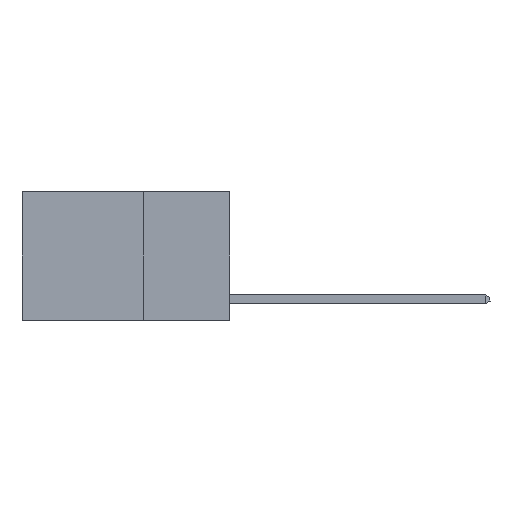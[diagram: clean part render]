
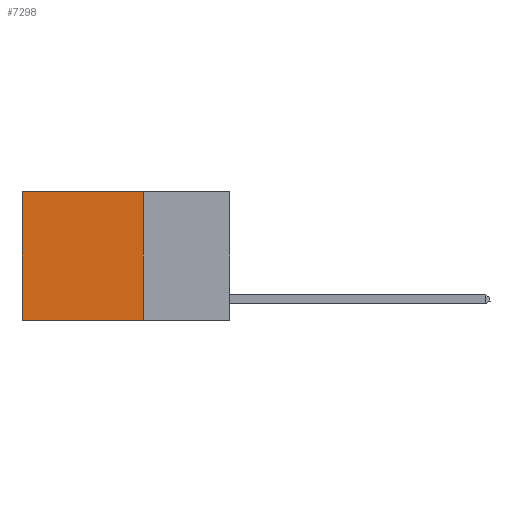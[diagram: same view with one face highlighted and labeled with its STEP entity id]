
A CAD part, left-side view. The second image highlights one B-rep face of the part: STEP entity #7298.
In plain terms, the highlighted planar face has unit normal (-1, 0, 0).
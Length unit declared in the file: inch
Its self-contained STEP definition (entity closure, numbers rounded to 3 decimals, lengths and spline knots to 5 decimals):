
#525 = EDGE_CURVE ( 'NONE', #13906, #12765, #7784, .T. ) ;
#599 = PLANE ( 'NONE',  #6531 ) ;
#750 = EDGE_CURVE ( 'NONE', #3400, #12765, #1172, .T. ) ;
#969 = VECTOR ( 'NONE', #12122, 39.37008 ) ;
#1172 = LINE ( 'NONE', #15113, #14037 ) ;
#1444 = EDGE_CURVE ( 'NONE', #3061, #13906, #5212, .T. ) ;
#1933 = DIRECTION ( 'NONE',  ( 1., 0., 0. ) ) ;
#2362 = VECTOR ( 'NONE', #7436, 39.37008 ) ;
#2688 = DIRECTION ( 'NONE',  ( 0., 0., -1. ) ) ;
#2980 = CARTESIAN_POINT ( 'NONE',  ( 0.2625, 0.6, 0. ) ) ;
#3061 = VERTEX_POINT ( 'NONE', #15967 ) ;
#3400 = VERTEX_POINT ( 'NONE', #2980 ) ;
#3490 = CARTESIAN_POINT ( 'NONE',  ( 0.2625, 0.6, -0.37 ) ) ;
#3659 = FACE_OUTER_BOUND ( 'NONE', #14649, .T. ) ;
#4446 = CARTESIAN_POINT ( 'NONE',  ( 0.2625, 0.25, -0.37 ) ) ;
#4913 = CARTESIAN_POINT ( 'NONE',  ( 0.2625, 0.25, 0. ) ) ;
#5131 = ORIENTED_EDGE ( 'NONE', *, *, #750, .T. ) ;
#5212 = LINE ( 'NONE', #10831, #14590 ) ;
#6531 = AXIS2_PLACEMENT_3D ( 'NONE', #9468, #1933, #10704 ) ;
#6574 = LINE ( 'NONE', #4913, #2362 ) ;
#6979 = ORIENTED_EDGE ( 'NONE', *, *, #525, .F. ) ;
#7298 = ADVANCED_FACE ( 'NONE', ( #3659 ), #599, .F. ) ;
#7436 = DIRECTION ( 'NONE',  ( 0., 1., 0. ) ) ;
#7784 = LINE ( 'NONE', #9748, #969 ) ;
#9055 = DIRECTION ( 'NONE',  ( 0., 0., -1. ) ) ;
#9468 = CARTESIAN_POINT ( 'NONE',  ( 0.2625, 0.25, 0. ) ) ;
#9748 = CARTESIAN_POINT ( 'NONE',  ( 0.2625, 0.25, -0.37 ) ) ;
#10459 = ORIENTED_EDGE ( 'NONE', *, *, #1444, .F. ) ;
#10704 = DIRECTION ( 'NONE',  ( 0., 0., -1. ) ) ;
#10831 = CARTESIAN_POINT ( 'NONE',  ( 0.2625, 0.25, 0. ) ) ;
#11013 = EDGE_CURVE ( 'NONE', #3061, #3400, #6574, .T. ) ;
#11533 = ORIENTED_EDGE ( 'NONE', *, *, #11013, .T. ) ;
#12122 = DIRECTION ( 'NONE',  ( 0., 1., 0. ) ) ;
#12765 = VERTEX_POINT ( 'NONE', #3490 ) ;
#13906 = VERTEX_POINT ( 'NONE', #4446 ) ;
#14037 = VECTOR ( 'NONE', #9055, 39.37008 ) ;
#14590 = VECTOR ( 'NONE', #2688, 39.37008 ) ;
#14649 = EDGE_LOOP ( 'NONE', ( #5131, #6979, #10459, #11533 ) ) ;
#15113 = CARTESIAN_POINT ( 'NONE',  ( 0.2625, 0.6, 0. ) ) ;
#15967 = CARTESIAN_POINT ( 'NONE',  ( 0.2625, 0.25, 0. ) ) ;
